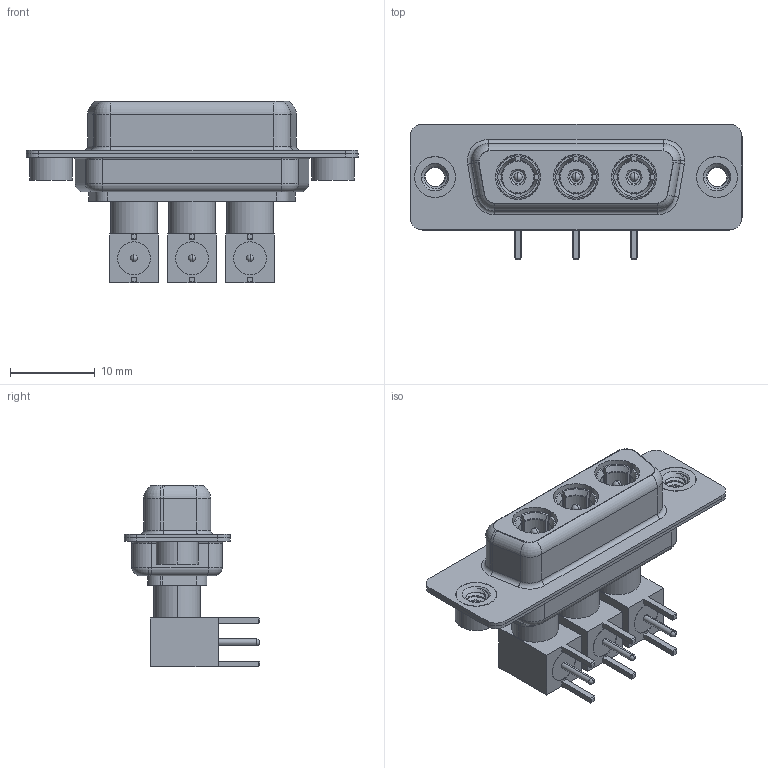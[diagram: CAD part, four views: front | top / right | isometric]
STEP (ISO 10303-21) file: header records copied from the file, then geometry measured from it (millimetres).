
FILE_DESCRIPTION (( 'STEP AP203' ), '1' );
FILE_NAME ('630-3W3-640-5T2.STEP', '2022-05-30T13:50:40', ( '' ), ( '' ), 'SwSTEP 2.0', 'SolidWorks 2020', '' );
FILE_SCHEMA (( 'CONFIG_CONTROL_DESIGN' ));
Length unit declared in the file: millimetre
Products named in the file (14): 630Combo Housing_3W3; Co-Ax Plug Assy_RA; 630Combo Shell Front_15 Contacts; Insulator Pin_Straight PC Tail; RA Back Shell; Co-Ax Plug_RA PC Tail; 630Combo Shell Rear_15 Contacts; 630Combo Threaded Rivet_2; Pin_RA; Insulator RA Pin; Locking Collar; 630-3W3-640-5T2
Assembly tree (26 placements, depth 3):
  630-3W3-640-5T2
    630Combo Housing_3W3
    630Combo Shell Front_15 Contacts
    630Combo Shell Rear_15 Contacts
    630Combo Threaded Rivet_2  x2
    Co-Ax Plug Assy_RA
      Co-Ax Plug_RA PC Tail
      Insulator Pin_Straight PC Tail
      Pin_RA
      Locking Collar
      RA Back Shell
      Insulator RA Pin
    Co-Ax Plug Assy_RA
      Co-Ax Plug_RA PC Tail
      Insulator Pin_Straight PC Tail
      Pin_RA
      Locking Collar
      RA Back Shell
      Insulator RA Pin
    Co-Ax Plug Assy_RA
      Co-Ax Plug_RA PC Tail
      Insulator Pin_Straight PC Tail
      Pin_RA
      Locking Collar
      RA Back Shell
      Insulator RA Pin
Bounding box: 39.2 x 16 x 21.41 mm (x, y, z)
Volume: 3140.5 mm3; surface area: 7789.5 mm2
Topology: 23 solids, 23 shells, 783 faces, 1888 edges, 1180 vertices
Faces by surface type: cylinder 332, plane 268, cone 87, torus 75, sphere 12, bspline 9
Entity records: 16007 total; most frequent: CARTESIAN_POINT 4013, DIRECTION 2290, ORIENTED_EDGE 2034, EDGE_CURVE 1017, AXIS2_PLACEMENT_3D 924, VERTEX_POINT 640, EDGE_LOOP 479, CIRCLE 472
